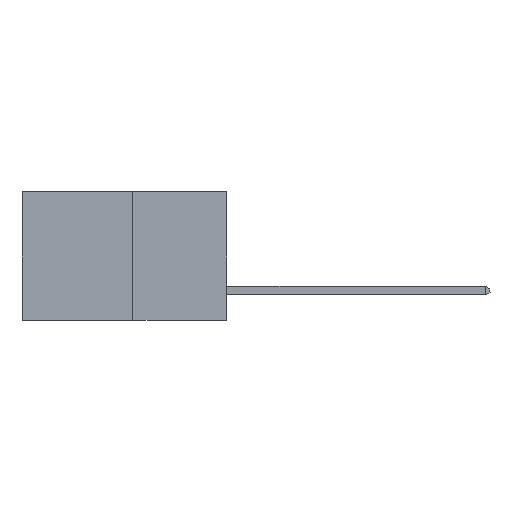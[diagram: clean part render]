
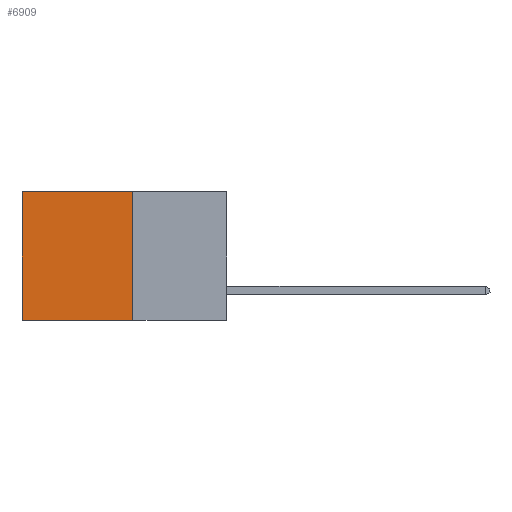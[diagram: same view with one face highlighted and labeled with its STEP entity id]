
A CAD part, left-side view. The second image highlights one B-rep face of the part: STEP entity #6909.
In plain terms, the highlighted planar face has unit normal (-1, 0, 0).
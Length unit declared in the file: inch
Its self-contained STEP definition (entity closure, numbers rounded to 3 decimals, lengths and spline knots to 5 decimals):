
#454 = AXIS2_PLACEMENT_3D ( 'NONE', #2360, #2313, #2288 ) ;
#622 = DIRECTION ( 'NONE',  ( 0., 0., -1. ) ) ;
#796 = VERTEX_POINT ( 'NONE', #5553 ) ;
#870 = DIRECTION ( 'NONE',  ( 0., 1., 0. ) ) ;
#935 = VERTEX_POINT ( 'NONE', #3807 ) ;
#1050 = CARTESIAN_POINT ( 'NONE',  ( 0.277, 0.27, -0.37 ) ) ;
#1085 = VECTOR ( 'NONE', #870, 39.37008 ) ;
#1234 = EDGE_CURVE ( 'NONE', #935, #5594, #2697, .T. ) ;
#1488 = LINE ( 'NONE', #3363, #10661 ) ;
#1660 = ORIENTED_EDGE ( 'NONE', *, *, #1234, .F. ) ;
#1675 = EDGE_CURVE ( 'NONE', #3178, #796, #7779, .T. ) ;
#2288 = DIRECTION ( 'NONE',  ( 0., 0., -1. ) ) ;
#2313 = DIRECTION ( 'NONE',  ( 1., 0., 0. ) ) ;
#2360 = CARTESIAN_POINT ( 'NONE',  ( 0.277, 0.27, -0.37 ) ) ;
#2391 = PLANE ( 'NONE',  #454 ) ;
#2409 = VECTOR ( 'NONE', #8409, 39.37008 ) ;
#2697 = LINE ( 'NONE', #9963, #2409 ) ;
#2999 = CARTESIAN_POINT ( 'NONE',  ( 0.277, 0.59, -0.37 ) ) ;
#3178 = VERTEX_POINT ( 'NONE', #4674 ) ;
#3363 = CARTESIAN_POINT ( 'NONE',  ( 0.277, 0.59, -0.37 ) ) ;
#3446 = DIRECTION ( 'NONE',  ( 0., 0., -1. ) ) ;
#3807 = CARTESIAN_POINT ( 'NONE',  ( 0.277, 0.27, -0.37 ) ) ;
#4674 = CARTESIAN_POINT ( 'NONE',  ( 0.277, 0.27, 0. ) ) ;
#4887 = CARTESIAN_POINT ( 'NONE',  ( 0.277, 0.27, 0. ) ) ;
#4944 = FACE_OUTER_BOUND ( 'NONE', #10934, .T. ) ;
#5553 = CARTESIAN_POINT ( 'NONE',  ( 0.277, 0.59, 0. ) ) ;
#5594 = VERTEX_POINT ( 'NONE', #2999 ) ;
#5689 = EDGE_CURVE ( 'NONE', #3178, #935, #10993, .T. ) ;
#6773 = EDGE_CURVE ( 'NONE', #796, #5594, #1488, .T. ) ;
#6909 = ADVANCED_FACE ( 'NONE', ( #4944 ), #2391, .F. ) ;
#7630 = ORIENTED_EDGE ( 'NONE', *, *, #1675, .T. ) ;
#7779 = LINE ( 'NONE', #4887, #1085 ) ;
#8056 = ORIENTED_EDGE ( 'NONE', *, *, #6773, .T. ) ;
#8409 = DIRECTION ( 'NONE',  ( 0., 1., 0. ) ) ;
#9079 = VECTOR ( 'NONE', #622, 39.37008 ) ;
#9963 = CARTESIAN_POINT ( 'NONE',  ( 0.277, 0.27, -0.37 ) ) ;
#10661 = VECTOR ( 'NONE', #3446, 39.37008 ) ;
#10934 = EDGE_LOOP ( 'NONE', ( #8056, #1660, #11313, #7630 ) ) ;
#10993 = LINE ( 'NONE', #1050, #9079 ) ;
#11313 = ORIENTED_EDGE ( 'NONE', *, *, #5689, .F. ) ;
